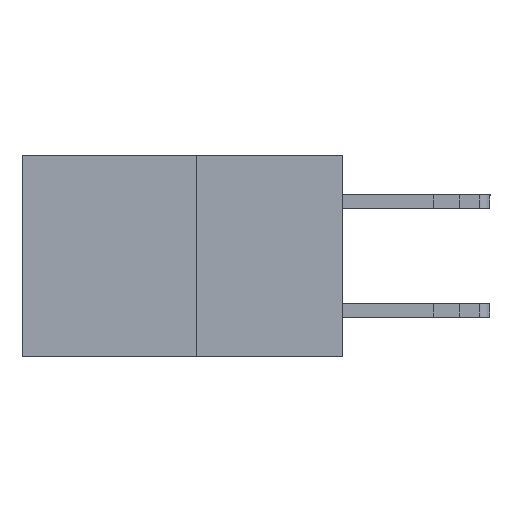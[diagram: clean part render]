
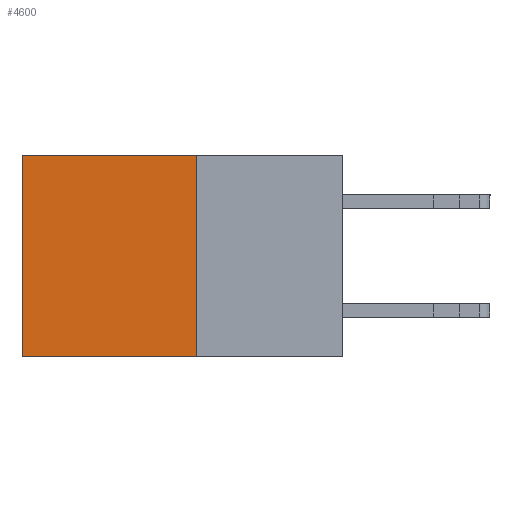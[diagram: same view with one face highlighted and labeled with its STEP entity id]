
A CAD part, left-side view. The second image highlights one B-rep face of the part: STEP entity #4600.
In plain terms, the highlighted planar face has unit normal (-1, 0, 0).
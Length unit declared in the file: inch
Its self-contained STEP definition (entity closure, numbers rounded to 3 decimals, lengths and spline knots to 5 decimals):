
#108 = VERTEX_POINT ( 'NONE', #5257 ) ;
#141 = CARTESIAN_POINT ( 'NONE',  ( 0.277, 0.27, -0.37 ) ) ;
#353 = LINE ( 'NONE', #3087, #2967 ) ;
#793 = EDGE_CURVE ( 'NONE', #4228, #2038, #353, .T. ) ;
#944 = LINE ( 'NONE', #4846, #6757 ) ;
#956 = VECTOR ( 'NONE', #3960, 39.37008 ) ;
#1258 = ORIENTED_EDGE ( 'NONE', *, *, #793, .F. ) ;
#2038 = VERTEX_POINT ( 'NONE', #6693 ) ;
#2735 = DIRECTION ( 'NONE',  ( 0., 0., -1. ) ) ;
#2967 = VECTOR ( 'NONE', #11173, 39.37008 ) ;
#3087 = CARTESIAN_POINT ( 'NONE',  ( 0.277, 0.27, -0.37 ) ) ;
#3340 = AXIS2_PLACEMENT_3D ( 'NONE', #6856, #6673, #6587 ) ;
#3960 = DIRECTION ( 'NONE',  ( 0., 1., 0. ) ) ;
#4228 = VERTEX_POINT ( 'NONE', #12184 ) ;
#4600 = ADVANCED_FACE ( 'NONE', ( #6223 ), #6835, .F. ) ;
#4846 = CARTESIAN_POINT ( 'NONE',  ( 0.277, 0.59, -0.37 ) ) ;
#5000 = VERTEX_POINT ( 'NONE', #7764 ) ;
#5022 = ORIENTED_EDGE ( 'NONE', *, *, #11874, .T. ) ;
#5257 = CARTESIAN_POINT ( 'NONE',  ( 0.277, 0.59, -0.37 ) ) ;
#5399 = ORIENTED_EDGE ( 'NONE', *, *, #11454, .T. ) ;
#6223 = FACE_OUTER_BOUND ( 'NONE', #9550, .T. ) ;
#6587 = DIRECTION ( 'NONE',  ( 0., 0., -1. ) ) ;
#6673 = DIRECTION ( 'NONE',  ( 1., 0., 0. ) ) ;
#6693 = CARTESIAN_POINT ( 'NONE',  ( 0.277, 0.27, -0.37 ) ) ;
#6757 = VECTOR ( 'NONE', #2735, 39.37008 ) ;
#6835 = PLANE ( 'NONE',  #3340 ) ;
#6856 = CARTESIAN_POINT ( 'NONE',  ( 0.277, 0.27, -0.37 ) ) ;
#7764 = CARTESIAN_POINT ( 'NONE',  ( 0.277, 0.59, 0. ) ) ;
#8868 = DIRECTION ( 'NONE',  ( 0., 1., 0. ) ) ;
#9550 = EDGE_LOOP ( 'NONE', ( #5022, #13762, #1258, #5399 ) ) ;
#10645 = LINE ( 'NONE', #141, #13120 ) ;
#11173 = DIRECTION ( 'NONE',  ( 0., 0., -1. ) ) ;
#11454 = EDGE_CURVE ( 'NONE', #4228, #5000, #12138, .T. ) ;
#11488 = CARTESIAN_POINT ( 'NONE',  ( 0.277, 0.27, 0. ) ) ;
#11874 = EDGE_CURVE ( 'NONE', #5000, #108, #944, .T. ) ;
#12138 = LINE ( 'NONE', #11488, #956 ) ;
#12184 = CARTESIAN_POINT ( 'NONE',  ( 0.277, 0.27, 0. ) ) ;
#12296 = EDGE_CURVE ( 'NONE', #2038, #108, #10645, .T. ) ;
#13120 = VECTOR ( 'NONE', #8868, 39.37008 ) ;
#13762 = ORIENTED_EDGE ( 'NONE', *, *, #12296, .F. ) ;
